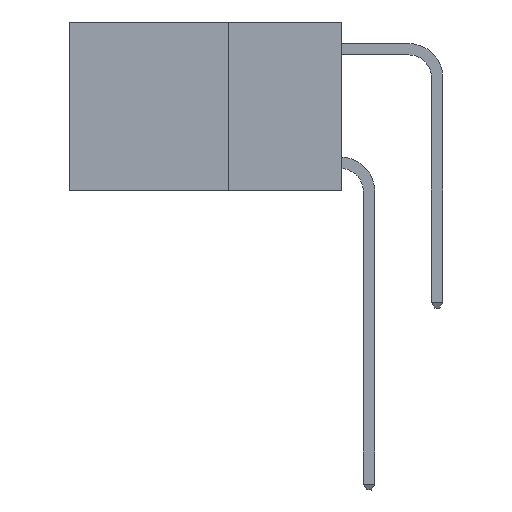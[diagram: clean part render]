
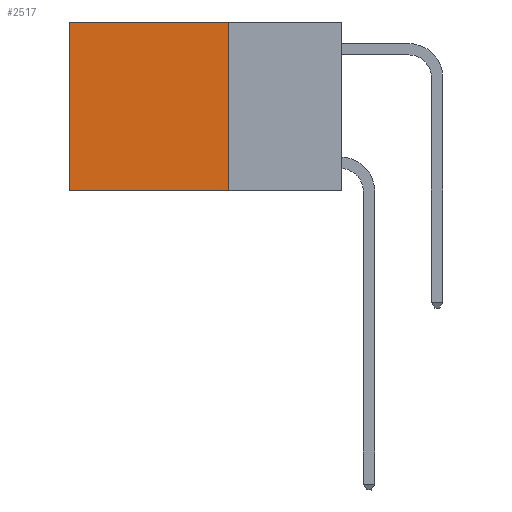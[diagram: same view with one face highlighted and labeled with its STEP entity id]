
A CAD part, left-side view. The second image highlights one B-rep face of the part: STEP entity #2517.
In plain terms, the highlighted planar face has unit normal (-1, 0, 0).
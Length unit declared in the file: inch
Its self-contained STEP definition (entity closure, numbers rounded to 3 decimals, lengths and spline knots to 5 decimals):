
#916 = ORIENTED_EDGE ( 'NONE', *, *, #7500, .F. ) ;
#1305 = ORIENTED_EDGE ( 'NONE', *, *, #9167, .F. ) ;
#2387 = AXIS2_PLACEMENT_3D ( 'NONE', #8280, #23034, #10398 ) ;
#2517 = ADVANCED_FACE ( 'NONE', ( #18558 ), #18796, .F. ) ;
#2742 = VECTOR ( 'NONE', #24218, 39.37008 ) ;
#4050 = EDGE_CURVE ( 'NONE', #11396, #4574, #8981, .T. ) ;
#4574 = VERTEX_POINT ( 'NONE', #6858 ) ;
#6858 = CARTESIAN_POINT ( 'NONE',  ( 0.2625, 0.6, -0.37 ) ) ;
#7500 = EDGE_CURVE ( 'NONE', #24406, #4574, #22656, .T. ) ;
#8280 = CARTESIAN_POINT ( 'NONE',  ( 0.2625, 0.25, 0. ) ) ;
#8747 = DIRECTION ( 'NONE',  ( 0., 1., 0. ) ) ;
#8981 = LINE ( 'NONE', #22118, #2742 ) ;
#9167 = EDGE_CURVE ( 'NONE', #27245, #24406, #16992, .T. ) ;
#9378 = CARTESIAN_POINT ( 'NONE',  ( 0.2625, 0.6, 0. ) ) ;
#10398 = DIRECTION ( 'NONE',  ( 0., 0., -1. ) ) ;
#11148 = CARTESIAN_POINT ( 'NONE',  ( 0.2625, 0.25, 0. ) ) ;
#11351 = VECTOR ( 'NONE', #14466, 39.37008 ) ;
#11396 = VERTEX_POINT ( 'NONE', #9378 ) ;
#12964 = CARTESIAN_POINT ( 'NONE',  ( 0.2625, 0.25, -0.37 ) ) ;
#13261 = DIRECTION ( 'NONE',  ( 0., 1., 0. ) ) ;
#14466 = DIRECTION ( 'NONE',  ( 0., 0., -1. ) ) ;
#15620 = ORIENTED_EDGE ( 'NONE', *, *, #16297, .T. ) ;
#16297 = EDGE_CURVE ( 'NONE', #27245, #11396, #19493, .T. ) ;
#16992 = LINE ( 'NONE', #20780, #11351 ) ;
#17036 = VECTOR ( 'NONE', #8747, 39.37008 ) ;
#17562 = EDGE_LOOP ( 'NONE', ( #27075, #916, #1305, #15620 ) ) ;
#18558 = FACE_OUTER_BOUND ( 'NONE', #17562, .T. ) ;
#18796 = PLANE ( 'NONE',  #2387 ) ;
#18975 = CARTESIAN_POINT ( 'NONE',  ( 0.2625, 0.25, 0. ) ) ;
#19493 = LINE ( 'NONE', #11148, #24415 ) ;
#20780 = CARTESIAN_POINT ( 'NONE',  ( 0.2625, 0.25, 0. ) ) ;
#20831 = CARTESIAN_POINT ( 'NONE',  ( 0.2625, 0.25, -0.37 ) ) ;
#22118 = CARTESIAN_POINT ( 'NONE',  ( 0.2625, 0.6, 0. ) ) ;
#22656 = LINE ( 'NONE', #12964, #17036 ) ;
#23034 = DIRECTION ( 'NONE',  ( 1., 0., 0. ) ) ;
#24218 = DIRECTION ( 'NONE',  ( 0., 0., -1. ) ) ;
#24406 = VERTEX_POINT ( 'NONE', #20831 ) ;
#24415 = VECTOR ( 'NONE', #13261, 39.37008 ) ;
#27075 = ORIENTED_EDGE ( 'NONE', *, *, #4050, .T. ) ;
#27245 = VERTEX_POINT ( 'NONE', #18975 ) ;
